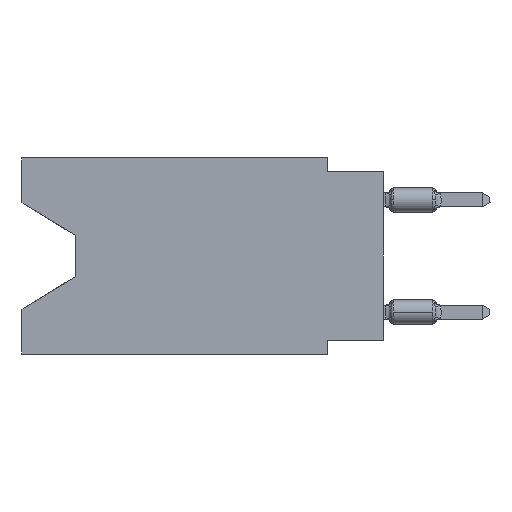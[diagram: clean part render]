
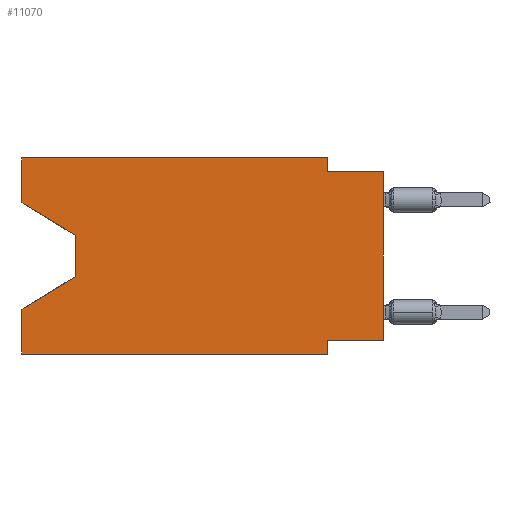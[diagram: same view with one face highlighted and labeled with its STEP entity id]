
A CAD part, left-side view. The second image highlights one B-rep face of the part: STEP entity #11070.
In plain terms, the highlighted planar face has unit normal (-1, 0, 0).
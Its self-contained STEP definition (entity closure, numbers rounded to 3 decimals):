
#532 = PLANE ( 'NONE',  #53610 ) ;
#747 = DIRECTION ( 'NONE',  ( 0., 0., 1. ) ) ;
#1301 = VECTOR ( 'NONE', #24080, 1000. ) ;
#1430 = VECTOR ( 'NONE', #51464, 1000. ) ;
#1580 = VERTEX_POINT ( 'NONE', #16842 ) ;
#1612 = CARTESIAN_POINT ( 'NONE',  ( 0., 13.97, -5.385 ) ) ;
#2515 = VECTOR ( 'NONE', #16161, 1000. ) ;
#3270 = CARTESIAN_POINT ( 'NONE',  ( 0., 2.54, -8.89 ) ) ;
#3439 = VERTEX_POINT ( 'NONE', #22438 ) ;
#5068 = ORIENTED_EDGE ( 'NONE', *, *, #14872, .T. ) ;
#5162 = VECTOR ( 'NONE', #20305, 1000. ) ;
#5337 = VERTEX_POINT ( 'NONE', #41617 ) ;
#6101 = CARTESIAN_POINT ( 'NONE',  ( 0., 0., -0.635 ) ) ;
#6435 = ORIENTED_EDGE ( 'NONE', *, *, #48937, .T. ) ;
#6514 = VERTEX_POINT ( 'NONE', #41401 ) ;
#6586 = DIRECTION ( 'NONE',  ( 0., 0.855, -0.519 ) ) ;
#6692 = CARTESIAN_POINT ( 'NONE',  ( 0., 16.383, 0. ) ) ;
#6955 = EDGE_CURVE ( 'NONE', #54806, #24467, #11127, .T. ) ;
#7541 = CARTESIAN_POINT ( 'NONE',  ( 0., 2.54, 0. ) ) ;
#8742 = CARTESIAN_POINT ( 'NONE',  ( 0., 2.54, 0. ) ) ;
#9379 = VERTEX_POINT ( 'NONE', #53119 ) ;
#9566 = ORIENTED_EDGE ( 'NONE', *, *, #22458, .F. ) ;
#10921 = ORIENTED_EDGE ( 'NONE', *, *, #41699, .T. ) ;
#11070 = ADVANCED_FACE ( 'NONE', ( #27911 ), #532, .F. ) ;
#11127 = LINE ( 'NONE', #6692, #1430 ) ;
#14872 = EDGE_CURVE ( 'NONE', #1580, #5337, #55773, .T. ) ;
#15322 = CARTESIAN_POINT ( 'NONE',  ( 0., 16.383, -8.89 ) ) ;
#15993 = VECTOR ( 'NONE', #6586, 1000. ) ;
#16161 = DIRECTION ( 'NONE',  ( 0., 0., 1. ) ) ;
#16322 = VERTEX_POINT ( 'NONE', #38197 ) ;
#16730 = EDGE_CURVE ( 'NONE', #1580, #56052, #53537, .T. ) ;
#16793 = DIRECTION ( 'NONE',  ( 0., 0., -1. ) ) ;
#16842 = CARTESIAN_POINT ( 'NONE',  ( 0., 0., -8.255 ) ) ;
#17025 = CARTESIAN_POINT ( 'NONE',  ( 0., 16.383, 0. ) ) ;
#17587 = LINE ( 'NONE', #8742, #50471 ) ;
#17899 = DIRECTION ( 'NONE',  ( 0., 0., -1. ) ) ;
#19292 = CARTESIAN_POINT ( 'NONE',  ( 0., 16.383, -2.038 ) ) ;
#19362 = ORIENTED_EDGE ( 'NONE', *, *, #37652, .T. ) ;
#19411 = ORIENTED_EDGE ( 'NONE', *, *, #45975, .F. ) ;
#20088 = ORIENTED_EDGE ( 'NONE', *, *, #6955, .F. ) ;
#20305 = DIRECTION ( 'NONE',  ( 0., -1., 0. ) ) ;
#20425 = CARTESIAN_POINT ( 'NONE',  ( 0., 0., 0. ) ) ;
#20809 = EDGE_CURVE ( 'NONE', #40330, #49579, #47660, .T. ) ;
#21773 = VECTOR ( 'NONE', #27855, 1000. ) ;
#22040 = CARTESIAN_POINT ( 'NONE',  ( 0., 0., -8.255 ) ) ;
#22044 = CARTESIAN_POINT ( 'NONE',  ( 0., 16.383, 0. ) ) ;
#22146 = CARTESIAN_POINT ( 'NONE',  ( 0., 16.383, -6.852 ) ) ;
#22438 = CARTESIAN_POINT ( 'NONE',  ( 0., 13.97, -3.505 ) ) ;
#22458 = EDGE_CURVE ( 'NONE', #37024, #5337, #46441, .T. ) ;
#22836 = LINE ( 'NONE', #58157, #53632 ) ;
#23235 = VECTOR ( 'NONE', #43539, 1000. ) ;
#24080 = DIRECTION ( 'NONE',  ( 0., -1., 0. ) ) ;
#24467 = VERTEX_POINT ( 'NONE', #7541 ) ;
#25577 = LINE ( 'NONE', #52062, #23235 ) ;
#25611 = CARTESIAN_POINT ( 'NONE',  ( 0., 16.383, -8.89 ) ) ;
#27154 = EDGE_CURVE ( 'NONE', #56052, #6514, #43618, .T. ) ;
#27855 = DIRECTION ( 'NONE',  ( 0., -0.855, -0.519 ) ) ;
#27911 = FACE_OUTER_BOUND ( 'NONE', #28319, .T. ) ;
#28319 = EDGE_LOOP ( 'NONE', ( #6435, #10921, #36561, #43726, #19362, #31727, #38276, #5068, #9566, #30034, #20088, #19411 ) ) ;
#30034 = ORIENTED_EDGE ( 'NONE', *, *, #33025, .F. ) ;
#31727 = ORIENTED_EDGE ( 'NONE', *, *, #27154, .F. ) ;
#33025 = EDGE_CURVE ( 'NONE', #24467, #37024, #17587, .T. ) ;
#34404 = VECTOR ( 'NONE', #16793, 1000. ) ;
#36561 = ORIENTED_EDGE ( 'NONE', *, *, #46180, .T. ) ;
#37024 = VERTEX_POINT ( 'NONE', #49343 ) ;
#37652 = EDGE_CURVE ( 'NONE', #40330, #6514, #42121, .T. ) ;
#38197 = CARTESIAN_POINT ( 'NONE',  ( 0., 13.97, -5.385 ) ) ;
#38276 = ORIENTED_EDGE ( 'NONE', *, *, #16730, .F. ) ;
#38714 = CARTESIAN_POINT ( 'NONE',  ( 0., 16.383, 0. ) ) ;
#40001 = DIRECTION ( 'NONE',  ( 0., 1., 0. ) ) ;
#40330 = VERTEX_POINT ( 'NONE', #25611 ) ;
#41401 = CARTESIAN_POINT ( 'NONE',  ( 0., 2.54, -8.89 ) ) ;
#41617 = CARTESIAN_POINT ( 'NONE',  ( 0., 0., -0.635 ) ) ;
#41699 = EDGE_CURVE ( 'NONE', #3439, #16322, #25577, .T. ) ;
#42121 = LINE ( 'NONE', #15322, #5162 ) ;
#43539 = DIRECTION ( 'NONE',  ( 0., 0., -1. ) ) ;
#43618 = LINE ( 'NONE', #3270, #34404 ) ;
#43726 = ORIENTED_EDGE ( 'NONE', *, *, #20809, .F. ) ;
#44678 = DIRECTION ( 'NONE',  ( 0., 0., -1. ) ) ;
#45975 = EDGE_CURVE ( 'NONE', #9379, #54806, #22836, .T. ) ;
#46180 = EDGE_CURVE ( 'NONE', #16322, #49579, #51358, .T. ) ;
#46182 = VECTOR ( 'NONE', #40001, 1000. ) ;
#46441 = LINE ( 'NONE', #6101, #1301 ) ;
#47223 = DIRECTION ( 'NONE',  ( 0., 0., 1. ) ) ;
#47422 = DIRECTION ( 'NONE',  ( 1., 0., 0. ) ) ;
#47660 = LINE ( 'NONE', #17025, #2515 ) ;
#48937 = EDGE_CURVE ( 'NONE', #9379, #3439, #50512, .T. ) ;
#49343 = CARTESIAN_POINT ( 'NONE',  ( 0., 2.54, -0.635 ) ) ;
#49579 = VERTEX_POINT ( 'NONE', #22146 ) ;
#50024 = CARTESIAN_POINT ( 'NONE',  ( 0., 2.54, -8.255 ) ) ;
#50471 = VECTOR ( 'NONE', #44678, 1000. ) ;
#50512 = LINE ( 'NONE', #19292, #21773 ) ;
#51358 = LINE ( 'NONE', #1612, #15993 ) ;
#51464 = DIRECTION ( 'NONE',  ( 0., -1., 0. ) ) ;
#52062 = CARTESIAN_POINT ( 'NONE',  ( 0., 13.97, -3.505 ) ) ;
#52647 = VECTOR ( 'NONE', #47223, 1000. ) ;
#53119 = CARTESIAN_POINT ( 'NONE',  ( 0., 16.383, -2.038 ) ) ;
#53537 = LINE ( 'NONE', #22040, #46182 ) ;
#53610 = AXIS2_PLACEMENT_3D ( 'NONE', #22044, #47422, #17899 ) ;
#53632 = VECTOR ( 'NONE', #747, 1000. ) ;
#54806 = VERTEX_POINT ( 'NONE', #38714 ) ;
#55773 = LINE ( 'NONE', #20425, #52647 ) ;
#56052 = VERTEX_POINT ( 'NONE', #50024 ) ;
#58157 = CARTESIAN_POINT ( 'NONE',  ( 0., 16.383, 0. ) ) ;
